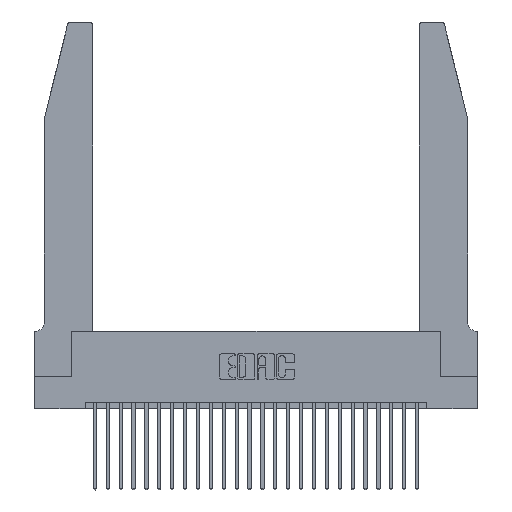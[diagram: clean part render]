
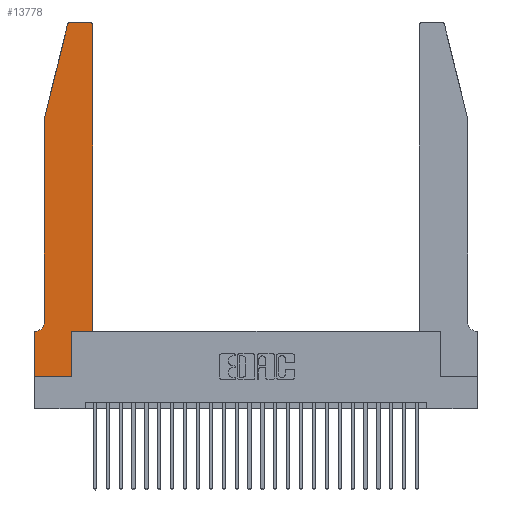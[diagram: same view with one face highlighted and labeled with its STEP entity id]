
A CAD part, top view. The second image highlights one B-rep face of the part: STEP entity #13778.
In plain terms, the highlighted planar face has unit normal (0, 0, 1).
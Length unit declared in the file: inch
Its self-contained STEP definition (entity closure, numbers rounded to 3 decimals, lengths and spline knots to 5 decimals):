
#34 = VECTOR ( 'NONE', #5517, 39.37008 ) ;
#98 = DIRECTION ( 'NONE',  ( 0., -1., 0. ) ) ;
#953 = DIRECTION ( 'NONE',  ( 1., 0., 0. ) ) ;
#1033 = LINE ( 'NONE', #11015, #19428 ) ;
#1131 = EDGE_CURVE ( 'NONE', #7227, #4957, #6057, .T. ) ;
#1163 = DIRECTION ( 'NONE',  ( 1., 0., 0. ) ) ;
#1229 = EDGE_CURVE ( 'NONE', #14116, #26327, #24845, .T. ) ;
#1242 = LINE ( 'NONE', #26329, #11078 ) ;
#1493 = AXIS2_PLACEMENT_3D ( 'NONE', #2751, #19609, #23856 ) ;
#2751 = CARTESIAN_POINT ( 'NONE',  ( 0.0055, 0.42, 0.37 ) ) ;
#3039 = CARTESIAN_POINT ( 'NONE',  ( 0.4205, 2.72, 0.37 ) ) ;
#3054 = ORIENTED_EDGE ( 'NONE', *, *, #17684, .T. ) ;
#3103 = CARTESIAN_POINT ( 'NONE',  ( 0.0755, 2., 0.37 ) ) ;
#3305 = LINE ( 'NONE', #3103, #14506 ) ;
#3327 = VECTOR ( 'NONE', #98, 39.37008 ) ;
#3466 = AXIS2_PLACEMENT_3D ( 'NONE', #5662, #26286, #9481 ) ;
#4314 = LINE ( 'NONE', #7478, #34 ) ;
#4379 = CARTESIAN_POINT ( 'NONE',  ( 0.2865, 0.35, 0.37 ) ) ;
#4957 = VERTEX_POINT ( 'NONE', #24164 ) ;
#5027 = DIRECTION ( 'NONE',  ( -1., 0., 0. ) ) ;
#5221 = EDGE_CURVE ( 'NONE', #17426, #14116, #24924, .T. ) ;
#5406 = ORIENTED_EDGE ( 'NONE', *, *, #1131, .T. ) ;
#5517 = DIRECTION ( 'NONE',  ( -0.239, -0.971, 0. ) ) ;
#5662 = CARTESIAN_POINT ( 'NONE',  ( 0., 0.35, 0.37 ) ) ;
#5808 = DIRECTION ( 'NONE',  ( 0., 1., 0. ) ) ;
#6057 = LINE ( 'NONE', #13255, #27182 ) ;
#6231 = EDGE_CURVE ( 'NONE', #22194, #8844, #27186, .T. ) ;
#7081 = VERTEX_POINT ( 'NONE', #25986 ) ;
#7227 = VERTEX_POINT ( 'NONE', #26294 ) ;
#7239 = CARTESIAN_POINT ( 'NONE',  ( 0.4505, 0.35, 0.37 ) ) ;
#7282 = ORIENTED_EDGE ( 'NONE', *, *, #9467, .T. ) ;
#7333 = CARTESIAN_POINT ( 'NONE',  ( 0., 0., 0.37 ) ) ;
#7384 = CARTESIAN_POINT ( 'NONE',  ( 0.284, 2.72, 0.37 ) ) ;
#7478 = CARTESIAN_POINT ( 'NONE',  ( 0.0755, 2., 0.37 ) ) ;
#8145 = FACE_OUTER_BOUND ( 'NONE', #10032, .T. ) ;
#8311 = PLANE ( 'NONE',  #3466 ) ;
#8681 = VECTOR ( 'NONE', #25584, 39.37008 ) ;
#8693 = DIRECTION ( 'NONE',  ( -1., 0., 0. ) ) ;
#8703 = CARTESIAN_POINT ( 'NONE',  ( 0.4205, 2.75, 0.37 ) ) ;
#8844 = VERTEX_POINT ( 'NONE', #27139 ) ;
#9467 = EDGE_CURVE ( 'NONE', #7081, #22940, #4314, .T. ) ;
#9481 = DIRECTION ( 'NONE',  ( 1., 0., 0. ) ) ;
#9809 = VERTEX_POINT ( 'NONE', #13792 ) ;
#10032 = EDGE_LOOP ( 'NONE', ( #23033, #10666, #7282, #17408, #24273, #5406, #3054, #26979, #19572, #26185, #11275, #24396 ) ) ;
#10133 = CARTESIAN_POINT ( 'NONE',  ( 0.4505, 0.35, 0.37 ) ) ;
#10666 = ORIENTED_EDGE ( 'NONE', *, *, #12831, .T. ) ;
#11015 = CARTESIAN_POINT ( 'NONE',  ( 0.2605, 2.75, 0.37 ) ) ;
#11078 = VECTOR ( 'NONE', #953, 39.37008 ) ;
#11275 = ORIENTED_EDGE ( 'NONE', *, *, #5221, .T. ) ;
#11353 = CIRCLE ( 'NONE', #1493, 0.07 ) ;
#12577 = EDGE_CURVE ( 'NONE', #9809, #17426, #1242, .T. ) ;
#12714 = VECTOR ( 'NONE', #5808, 39.37008 ) ;
#12803 = CARTESIAN_POINT ( 'NONE',  ( 0.0755, 2., 0.37 ) ) ;
#12831 = EDGE_CURVE ( 'NONE', #23975, #7081, #15016, .T. ) ;
#13255 = CARTESIAN_POINT ( 'NONE',  ( 0.0755, 0.35, 0.37 ) ) ;
#13756 = DIRECTION ( 'NONE',  ( 0., 0., 1. ) ) ;
#13778 = ADVANCED_FACE ( 'NONE', ( #8145 ), #8311, .T. ) ;
#13792 = CARTESIAN_POINT ( 'NONE',  ( 0.2865, 0.35, 0.37 ) ) ;
#14116 = VERTEX_POINT ( 'NONE', #23279 ) ;
#14506 = VECTOR ( 'NONE', #24336, 39.37008 ) ;
#15016 = CIRCLE ( 'NONE', #22156, 0.03 ) ;
#15658 = DIRECTION ( 'NONE',  ( 0., 0., 1. ) ) ;
#17408 = ORIENTED_EDGE ( 'NONE', *, *, #17976, .T. ) ;
#17413 = CARTESIAN_POINT ( 'NONE',  ( 0., 0., 0.37 ) ) ;
#17426 = VERTEX_POINT ( 'NONE', #7239 ) ;
#17684 = EDGE_CURVE ( 'NONE', #4957, #22194, #25108, .T. ) ;
#17693 = DIRECTION ( 'NONE',  ( 1., 0., 0. ) ) ;
#17976 = EDGE_CURVE ( 'NONE', #22940, #22239, #3305, .T. ) ;
#19080 = CARTESIAN_POINT ( 'NONE',  ( 0.0755, 0.42, 0.37 ) ) ;
#19293 = AXIS2_PLACEMENT_3D ( 'NONE', #3039, #13756, #17693 ) ;
#19428 = VECTOR ( 'NONE', #5027, 39.37008 ) ;
#19521 = VECTOR ( 'NONE', #1163, 39.37008 ) ;
#19572 = ORIENTED_EDGE ( 'NONE', *, *, #21640, .T. ) ;
#19609 = DIRECTION ( 'NONE',  ( 0., 0., -1. ) ) ;
#20028 = CARTESIAN_POINT ( 'NONE',  ( 0., 0., 0.37 ) ) ;
#20619 = EDGE_CURVE ( 'NONE', #22239, #7227, #11353, .T. ) ;
#21640 = EDGE_CURVE ( 'NONE', #8844, #9809, #23188, .T. ) ;
#21717 = CARTESIAN_POINT ( 'NONE',  ( 0.284, 2.75, 0.37 ) ) ;
#22108 = DIRECTION ( 'NONE',  ( 1., 0., 0. ) ) ;
#22156 = AXIS2_PLACEMENT_3D ( 'NONE', #7384, #15658, #22108 ) ;
#22194 = VERTEX_POINT ( 'NONE', #20028 ) ;
#22239 = VERTEX_POINT ( 'NONE', #19080 ) ;
#22940 = VERTEX_POINT ( 'NONE', #12803 ) ;
#23033 = ORIENTED_EDGE ( 'NONE', *, *, #23871, .T. ) ;
#23188 = LINE ( 'NONE', #4379, #8681 ) ;
#23279 = CARTESIAN_POINT ( 'NONE',  ( 0.4505, 2.72, 0.37 ) ) ;
#23856 = DIRECTION ( 'NONE',  ( -1., 0., 0. ) ) ;
#23871 = EDGE_CURVE ( 'NONE', #26327, #23975, #1033, .T. ) ;
#23975 = VERTEX_POINT ( 'NONE', #21717 ) ;
#24164 = CARTESIAN_POINT ( 'NONE',  ( 0., 0.35, 0.37 ) ) ;
#24273 = ORIENTED_EDGE ( 'NONE', *, *, #20619, .T. ) ;
#24336 = DIRECTION ( 'NONE',  ( 0., -1., 0. ) ) ;
#24396 = ORIENTED_EDGE ( 'NONE', *, *, #1229, .T. ) ;
#24845 = CIRCLE ( 'NONE', #19293, 0.03 ) ;
#24924 = LINE ( 'NONE', #10133, #12714 ) ;
#25108 = LINE ( 'NONE', #17413, #3327 ) ;
#25584 = DIRECTION ( 'NONE',  ( 0., 1., 0. ) ) ;
#25986 = CARTESIAN_POINT ( 'NONE',  ( 0.25487, 2.72718, 0.37 ) ) ;
#26185 = ORIENTED_EDGE ( 'NONE', *, *, #12577, .T. ) ;
#26286 = DIRECTION ( 'NONE',  ( 0., 0., 1. ) ) ;
#26294 = CARTESIAN_POINT ( 'NONE',  ( 0.0055, 0.35, 0.37 ) ) ;
#26327 = VERTEX_POINT ( 'NONE', #8703 ) ;
#26329 = CARTESIAN_POINT ( 'NONE',  ( 0.4505, 0.35, 0.37 ) ) ;
#26979 = ORIENTED_EDGE ( 'NONE', *, *, #6231, .T. ) ;
#27139 = CARTESIAN_POINT ( 'NONE',  ( 0.2865, 0., 0.37 ) ) ;
#27182 = VECTOR ( 'NONE', #8693, 39.37008 ) ;
#27186 = LINE ( 'NONE', #7333, #19521 ) ;
